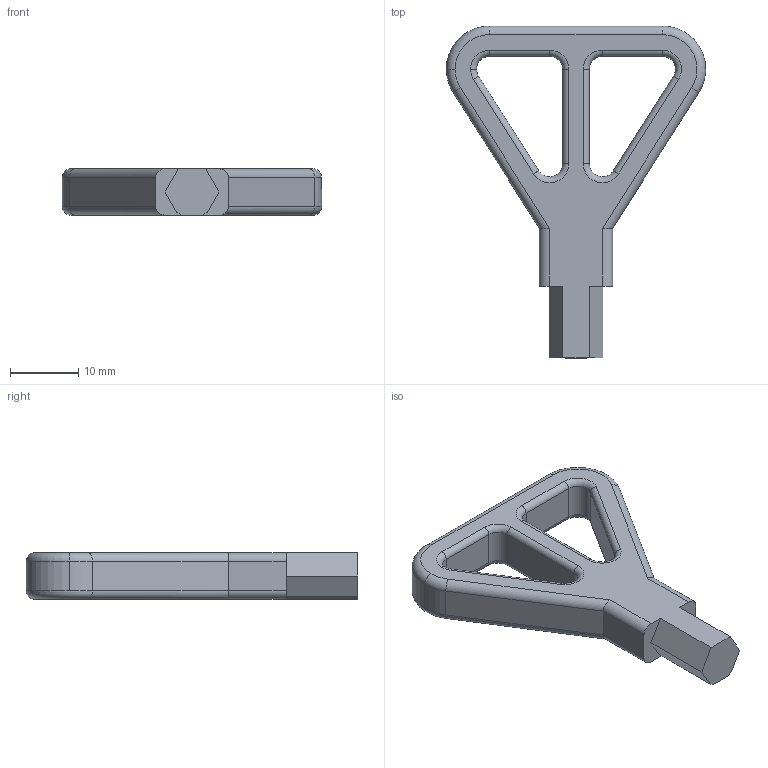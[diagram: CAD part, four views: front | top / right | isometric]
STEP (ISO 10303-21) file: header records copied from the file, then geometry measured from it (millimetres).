
FILE_DESCRIPTION (( 'STEP AP203' ), '1' );
FILE_NAME ('AF-HF-BT-PRT-001-STEP.STEP', '2020-10-30T17:23:08', ( '' ), ( '' ), 'SwSTEP 2.0', 'SolidWorks 2018', '' );
FILE_SCHEMA (( 'CONFIG_CONTROL_DESIGN' ));
Length unit declared in the file: inch
Products named in the file (1): AF-HF-BT-PRT-001-STEP
Bounding box: 38.1 x 48.77 x 6.83 mm (x, y, z)
Volume: 4525.9 mm3; surface area: 2845.3 mm2
Topology: 1 solids, 1 shells, 74 faces, 178 edges, 106 vertices
Faces by surface type: cylinder 28, plane 22, torus 20, bspline 4
Entity records: 2235 total; most frequent: CARTESIAN_POINT 411, DIRECTION 390, ORIENTED_EDGE 356, EDGE_CURVE 178, AXIS2_PLACEMENT_3D 149, VERTEX_POINT 106, VECTOR 92, LINE 92
